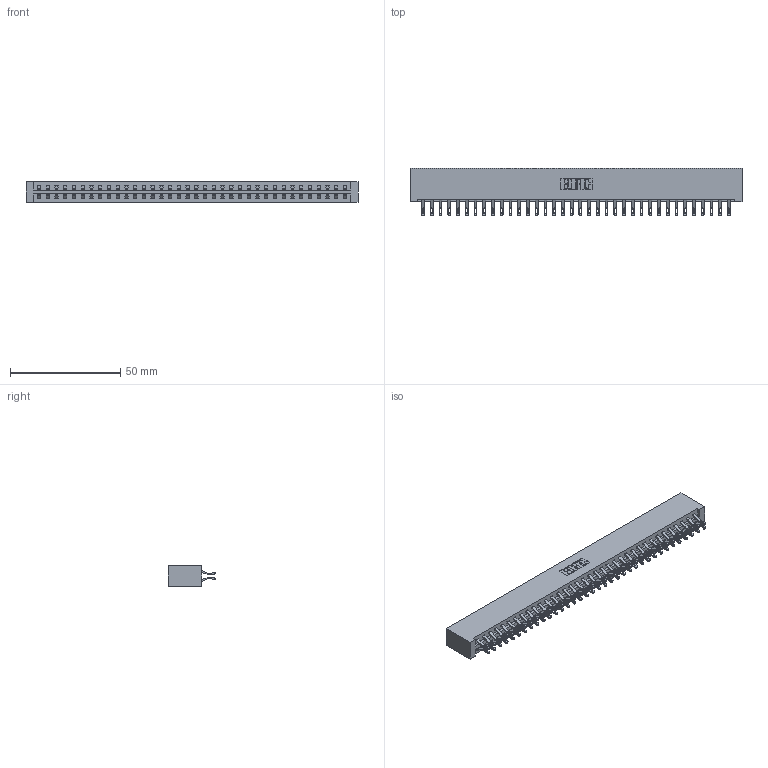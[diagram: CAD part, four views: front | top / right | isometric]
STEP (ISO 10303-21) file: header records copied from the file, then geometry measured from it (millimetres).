
FILE_DESCRIPTION (( 'STEP AP203' ), '1' );
FILE_NAME ('387-072-555-201.STEP', '2018-09-22T18:36:17', ( '' ), ( '' ), 'SwSTEP 2.0', 'SolidWorks 2016', '' );
FILE_SCHEMA (( 'CONFIG_CONTROL_DESIGN' ));
Length unit declared in the file: inch
Products named in the file (3): 337 Part_No Mounting Lugs; 345-292-001_555 Tail; 387-072-555-201
Assembly tree (73 placements, depth 2):
  387-072-555-201
    337 Part_No Mounting Lugs
    345-292-001_555 Tail  x72
Bounding box: 150.52 x 21.47 x 9.4 mm (x, y, z)
Volume: 16752.7 mm3; surface area: 19723.8 mm2
Topology: 73 solids, 73 shells, 4426 faces, 13895 edges, 9262 vertices
Faces by surface type: plane 2658, cylinder 1768
Entity records: 28737 total; most frequent: CARTESIAN_POINT 4880, ORIENTED_EDGE 4786, DIRECTION 4125, EDGE_CURVE 2393, VECTOR 2253, LINE 2253, VERTEX_POINT 1594, AXIS2_PLACEMENT_3D 936
